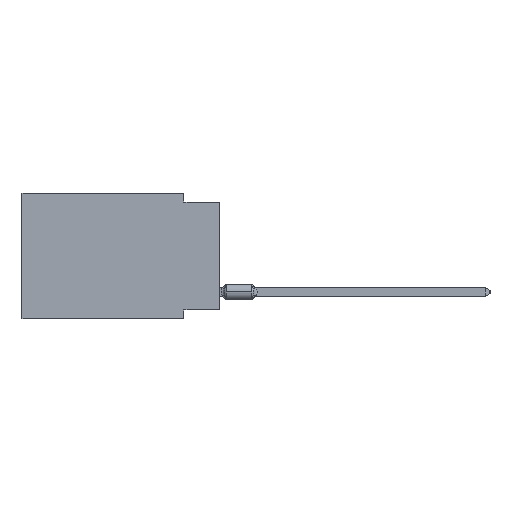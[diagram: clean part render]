
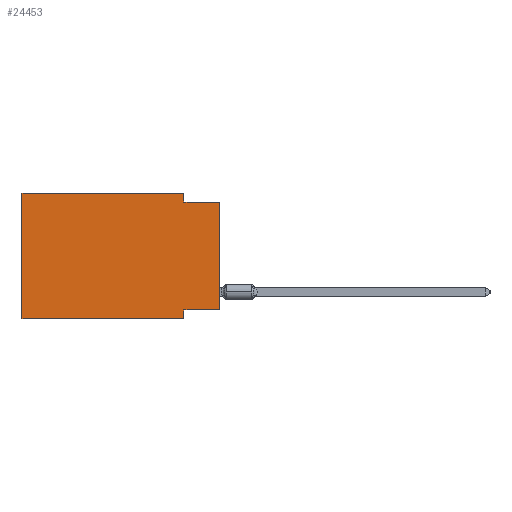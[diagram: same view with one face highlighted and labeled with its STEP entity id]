
A CAD part, left-side view. The second image highlights one B-rep face of the part: STEP entity #24453.
In plain terms, the highlighted planar face has unit normal (-1, 0, 0).
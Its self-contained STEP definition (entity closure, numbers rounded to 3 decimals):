
#48 = PLANE ( 'NONE',  #52490 ) ;
#1080 = VECTOR ( 'NONE', #51674, 1000. ) ;
#1927 = CARTESIAN_POINT ( 'NONE',  ( 0., 2.54, -8.255 ) ) ;
#2636 = LINE ( 'NONE', #17015, #1080 ) ;
#3282 = VERTEX_POINT ( 'NONE', #29214 ) ;
#3402 = CARTESIAN_POINT ( 'NONE',  ( 0., 2.54, -0.635 ) ) ;
#3556 = VERTEX_POINT ( 'NONE', #60667 ) ;
#4275 = CARTESIAN_POINT ( 'NONE',  ( 0., 13.97, -8.89 ) ) ;
#4904 = CARTESIAN_POINT ( 'NONE',  ( 0., 0., 0. ) ) ;
#5007 = CARTESIAN_POINT ( 'NONE',  ( 0., 13.97, 0. ) ) ;
#7884 = LINE ( 'NONE', #35337, #63102 ) ;
#8035 = ORIENTED_EDGE ( 'NONE', *, *, #78892, .F. ) ;
#11349 = ORIENTED_EDGE ( 'NONE', *, *, #19533, .F. ) ;
#13574 = EDGE_CURVE ( 'NONE', #62464, #60945, #14129, .T. ) ;
#14129 = LINE ( 'NONE', #71701, #20357 ) ;
#16624 = DIRECTION ( 'NONE',  ( 0., 0., 1. ) ) ;
#17015 = CARTESIAN_POINT ( 'NONE',  ( 0., 13.97, 0. ) ) ;
#17338 = DIRECTION ( 'NONE',  ( 0., -1., 0. ) ) ;
#17346 = VECTOR ( 'NONE', #42677, 1000. ) ;
#19533 = EDGE_CURVE ( 'NONE', #48622, #82556, #30061, .T. ) ;
#19880 = VECTOR ( 'NONE', #16624, 1000. ) ;
#20075 = VECTOR ( 'NONE', #17338, 1000. ) ;
#20357 = VECTOR ( 'NONE', #57750, 1000. ) ;
#23380 = LINE ( 'NONE', #4904, #19880 ) ;
#24453 = ADVANCED_FACE ( 'NONE', ( #75231 ), #48, .F. ) ;
#27063 = DIRECTION ( 'NONE',  ( 1., 0., 0. ) ) ;
#27478 = VECTOR ( 'NONE', #62914, 1000. ) ;
#27551 = LINE ( 'NONE', #55014, #76816 ) ;
#28028 = EDGE_CURVE ( 'NONE', #65277, #3556, #23380, .T. ) ;
#28810 = ORIENTED_EDGE ( 'NONE', *, *, #87057, .F. ) ;
#29214 = CARTESIAN_POINT ( 'NONE',  ( 0., 2.54, -8.89 ) ) ;
#30061 = LINE ( 'NONE', #55772, #17346 ) ;
#30542 = EDGE_LOOP ( 'NONE', ( #83136, #8035, #57125, #74109, #11349, #62933, #52561, #28810 ) ) ;
#35337 = CARTESIAN_POINT ( 'NONE',  ( 0., 0., -0.635 ) ) ;
#38033 = LINE ( 'NONE', #4275, #20075 ) ;
#39890 = EDGE_CURVE ( 'NONE', #74491, #3282, #46734, .T. ) ;
#39983 = CARTESIAN_POINT ( 'NONE',  ( 0., 2.54, -8.89 ) ) ;
#39988 = CARTESIAN_POINT ( 'NONE',  ( 0., 0., -8.255 ) ) ;
#40997 = DIRECTION ( 'NONE',  ( 0., 0., -1. ) ) ;
#42677 = DIRECTION ( 'NONE',  ( 0., 0., 1. ) ) ;
#46734 = LINE ( 'NONE', #39983, #27478 ) ;
#48622 = VERTEX_POINT ( 'NONE', #86126 ) ;
#51674 = DIRECTION ( 'NONE',  ( 0., -1., 0. ) ) ;
#52490 = AXIS2_PLACEMENT_3D ( 'NONE', #5007, #27063, #40997 ) ;
#52561 = ORIENTED_EDGE ( 'NONE', *, *, #39890, .F. ) ;
#55014 = CARTESIAN_POINT ( 'NONE',  ( 0., 0., -8.255 ) ) ;
#55772 = CARTESIAN_POINT ( 'NONE',  ( 0., 13.97, 0. ) ) ;
#57125 = ORIENTED_EDGE ( 'NONE', *, *, #13574, .F. ) ;
#57750 = DIRECTION ( 'NONE',  ( 0., 0., -1. ) ) ;
#59809 = EDGE_CURVE ( 'NONE', #48622, #3282, #38033, .T. ) ;
#60667 = CARTESIAN_POINT ( 'NONE',  ( 0., 0., -0.635 ) ) ;
#60945 = VERTEX_POINT ( 'NONE', #3402 ) ;
#61921 = DIRECTION ( 'NONE',  ( 0., -1., 0. ) ) ;
#62464 = VERTEX_POINT ( 'NONE', #69543 ) ;
#62914 = DIRECTION ( 'NONE',  ( 0., 0., -1. ) ) ;
#62933 = ORIENTED_EDGE ( 'NONE', *, *, #59809, .T. ) ;
#63102 = VECTOR ( 'NONE', #61921, 1000. ) ;
#65277 = VERTEX_POINT ( 'NONE', #39988 ) ;
#69543 = CARTESIAN_POINT ( 'NONE',  ( 0., 2.54, 0. ) ) ;
#70428 = EDGE_CURVE ( 'NONE', #82556, #62464, #2636, .T. ) ;
#71701 = CARTESIAN_POINT ( 'NONE',  ( 0., 2.54, 0. ) ) ;
#74109 = ORIENTED_EDGE ( 'NONE', *, *, #70428, .F. ) ;
#74491 = VERTEX_POINT ( 'NONE', #1927 ) ;
#75231 = FACE_OUTER_BOUND ( 'NONE', #30542, .T. ) ;
#76816 = VECTOR ( 'NONE', #82462, 1000. ) ;
#78253 = CARTESIAN_POINT ( 'NONE',  ( 0., 13.97, 0. ) ) ;
#78892 = EDGE_CURVE ( 'NONE', #60945, #3556, #7884, .T. ) ;
#82462 = DIRECTION ( 'NONE',  ( 0., 1., 0. ) ) ;
#82556 = VERTEX_POINT ( 'NONE', #78253 ) ;
#83136 = ORIENTED_EDGE ( 'NONE', *, *, #28028, .T. ) ;
#86126 = CARTESIAN_POINT ( 'NONE',  ( 0., 13.97, -8.89 ) ) ;
#87057 = EDGE_CURVE ( 'NONE', #65277, #74491, #27551, .T. ) ;
